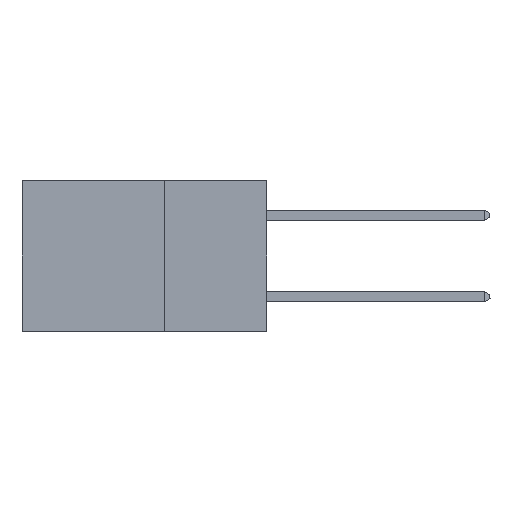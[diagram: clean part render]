
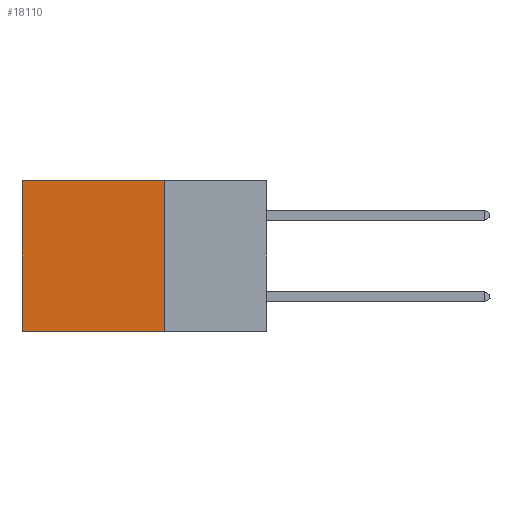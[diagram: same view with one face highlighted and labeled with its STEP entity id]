
A CAD part, left-side view. The second image highlights one B-rep face of the part: STEP entity #18110.
In plain terms, the highlighted planar face has unit normal (-1, 0, 0).
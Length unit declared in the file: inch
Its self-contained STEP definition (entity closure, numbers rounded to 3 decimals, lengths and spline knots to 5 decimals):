
#485 = LINE ( 'NONE', #1311, #18203 ) ;
#710 = ORIENTED_EDGE ( 'NONE', *, *, #7674, .F. ) ;
#1311 = CARTESIAN_POINT ( 'NONE',  ( 0.2875, 0.25, -0.37 ) ) ;
#2049 = LINE ( 'NONE', #6778, #24104 ) ;
#2940 = CARTESIAN_POINT ( 'NONE',  ( 0.2875, 0.25, 0. ) ) ;
#3225 = VERTEX_POINT ( 'NONE', #7061 ) ;
#4098 = VECTOR ( 'NONE', #17704, 39.37008 ) ;
#4564 = DIRECTION ( 'NONE',  ( 1., 0., 0. ) ) ;
#4658 = VERTEX_POINT ( 'NONE', #16098 ) ;
#6739 = CARTESIAN_POINT ( 'NONE',  ( 0.2875, 0.25, 0. ) ) ;
#6778 = CARTESIAN_POINT ( 'NONE',  ( 0.2875, 0.6, 0. ) ) ;
#7035 = DIRECTION ( 'NONE',  ( 0., 1., 0. ) ) ;
#7061 = CARTESIAN_POINT ( 'NONE',  ( 0.2875, 0.25, -0.37 ) ) ;
#7674 = EDGE_CURVE ( 'NONE', #3225, #14666, #485, .T. ) ;
#10671 = DIRECTION ( 'NONE',  ( 0., 1., 0. ) ) ;
#11330 = EDGE_CURVE ( 'NONE', #23038, #4658, #12075, .T. ) ;
#12075 = LINE ( 'NONE', #25874, #20735 ) ;
#12588 = ORIENTED_EDGE ( 'NONE', *, *, #11330, .T. ) ;
#14175 = FACE_OUTER_BOUND ( 'NONE', #15583, .T. ) ;
#14666 = VERTEX_POINT ( 'NONE', #22801 ) ;
#14769 = ORIENTED_EDGE ( 'NONE', *, *, #14794, .F. ) ;
#14794 = EDGE_CURVE ( 'NONE', #23038, #3225, #21179, .T. ) ;
#15583 = EDGE_LOOP ( 'NONE', ( #22761, #710, #14769, #12588 ) ) ;
#16098 = CARTESIAN_POINT ( 'NONE',  ( 0.2875, 0.6, 0. ) ) ;
#17573 = PLANE ( 'NONE',  #23895 ) ;
#17704 = DIRECTION ( 'NONE',  ( 0., 0., -1. ) ) ;
#18110 = ADVANCED_FACE ( 'NONE', ( #14175 ), #17573, .F. ) ;
#18203 = VECTOR ( 'NONE', #7035, 39.37008 ) ;
#19404 = EDGE_CURVE ( 'NONE', #4658, #14666, #2049, .T. ) ;
#19455 = DIRECTION ( 'NONE',  ( 0., 0., -1. ) ) ;
#19508 = DIRECTION ( 'NONE',  ( 0., 0., -1. ) ) ;
#20735 = VECTOR ( 'NONE', #10671, 39.37008 ) ;
#20937 = CARTESIAN_POINT ( 'NONE',  ( 0.2875, 0.25, 0. ) ) ;
#21179 = LINE ( 'NONE', #2940, #4098 ) ;
#22761 = ORIENTED_EDGE ( 'NONE', *, *, #19404, .T. ) ;
#22801 = CARTESIAN_POINT ( 'NONE',  ( 0.2875, 0.6, -0.37 ) ) ;
#23038 = VERTEX_POINT ( 'NONE', #20937 ) ;
#23895 = AXIS2_PLACEMENT_3D ( 'NONE', #6739, #4564, #19508 ) ;
#24104 = VECTOR ( 'NONE', #19455, 39.37008 ) ;
#25874 = CARTESIAN_POINT ( 'NONE',  ( 0.2875, 0.25, 0. ) ) ;
